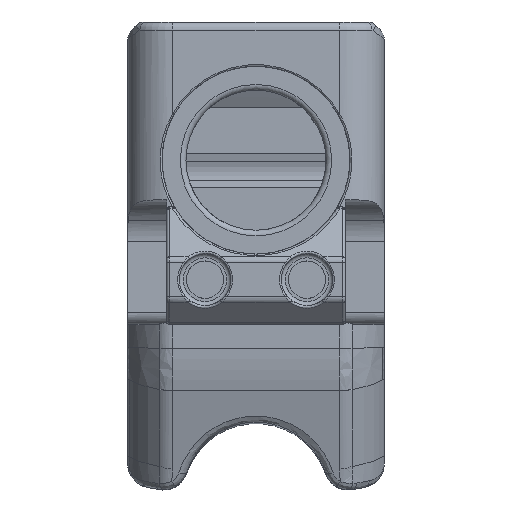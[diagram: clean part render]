
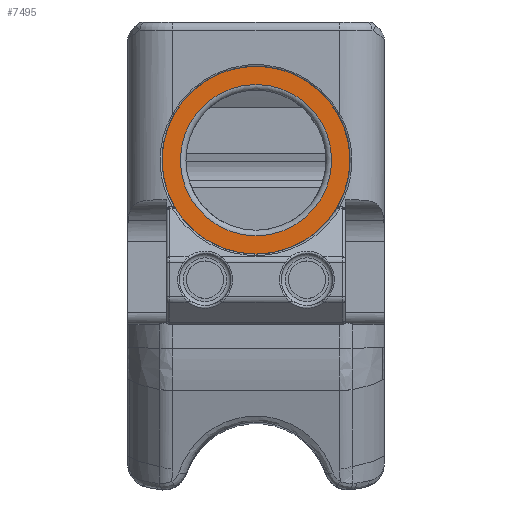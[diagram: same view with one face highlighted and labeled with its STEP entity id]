
A CAD part, front view. The second image highlights one B-rep face of the part: STEP entity #7495.
In plain terms, the highlighted planar face has unit normal (0, -1, 0).
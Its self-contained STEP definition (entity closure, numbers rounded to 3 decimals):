
#68=FACE_BOUND('',#1961,.T.);
#175=PLANE('',#8013);
#1480=FACE_OUTER_BOUND('',#1960,.T.);
#1960=EDGE_LOOP('',(#5120));
#1961=EDGE_LOOP('',(#5121));
#2461=CIRCLE('',#8006,9.425);
#2466=CIRCLE('',#8014,11.697);
#3147=VERTEX_POINT('',#11487);
#3160=VERTEX_POINT('',#11863);
#3875=EDGE_CURVE('',#3147,#3147,#2461,.T.);
#3896=EDGE_CURVE('',#3160,#3160,#2466,.T.);
#5120=ORIENTED_EDGE('',*,*,#3896,.T.);
#5121=ORIENTED_EDGE('',*,*,#3875,.F.);
#7495=ADVANCED_FACE('',(#1480,#68),#175,.T.);
#8006=AXIS2_PLACEMENT_3D('',#11488,#8948,#8949);
#8013=AXIS2_PLACEMENT_3D('',#11862,#8963,#8964);
#8014=AXIS2_PLACEMENT_3D('',#11864,#8965,#8966);
#8948=DIRECTION('center_axis',(0.,-1.,0.));
#8949=DIRECTION('ref_axis',(0.922,0.,0.388));
#8963=DIRECTION('center_axis',(0.,-1.,0.));
#8964=DIRECTION('ref_axis',(1.,0.,0.));
#8965=DIRECTION('center_axis',(0.,-1.,0.));
#8966=DIRECTION('ref_axis',(1.,0.,0.));
#11487=CARTESIAN_POINT('',(15.977,-18.733,-125.541));
#11488=CARTESIAN_POINT('Origin',(15.977,-18.733,-116.116));
#11862=CARTESIAN_POINT('Origin',(15.977,-18.733,-116.116));
#11863=CARTESIAN_POINT('',(15.977,-18.733,-127.813));
#11864=CARTESIAN_POINT('Origin',(15.977,-18.733,-116.116));
